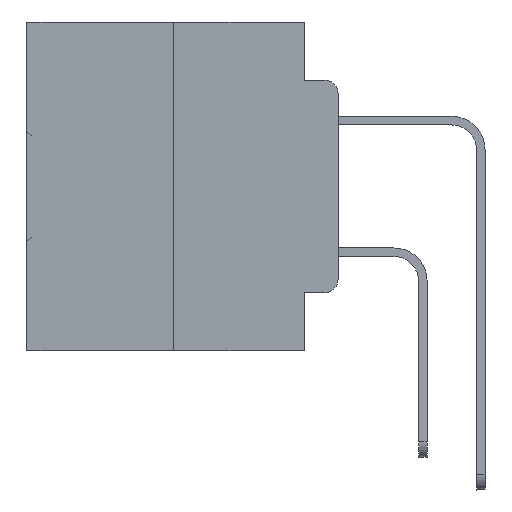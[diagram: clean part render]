
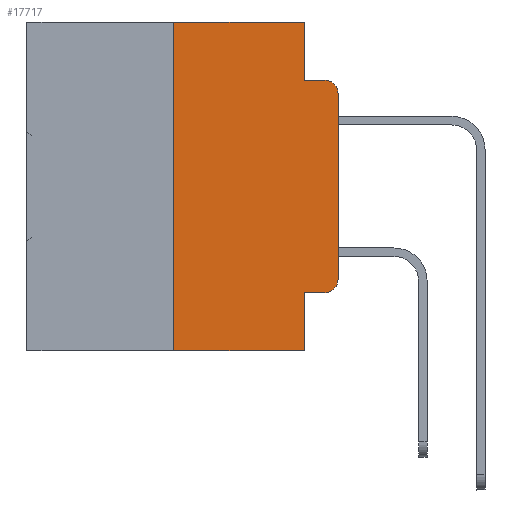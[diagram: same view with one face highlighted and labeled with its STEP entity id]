
A CAD part, left-side view. The second image highlights one B-rep face of the part: STEP entity #17717.
In plain terms, the highlighted planar face has unit normal (-1, 0, 0).
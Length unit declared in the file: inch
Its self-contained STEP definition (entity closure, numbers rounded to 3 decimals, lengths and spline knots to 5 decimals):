
#127 = CARTESIAN_POINT ( 'NONE',  ( 0., 0., -0.1085 ) ) ;
#275 = CARTESIAN_POINT ( 'NONE',  ( 0., 0., -0.3915 ) ) ;
#733 = VERTEX_POINT ( 'NONE', #14793 ) ;
#1035 = EDGE_CURVE ( 'NONE', #28705, #18398, #30167, .T. ) ;
#1122 = CARTESIAN_POINT ( 'NONE',  ( 0., 0.02, -0.4115 ) ) ;
#2019 = ORIENTED_EDGE ( 'NONE', *, *, #21079, .T. ) ;
#2238 = DIRECTION ( 'NONE',  ( 0., -1., 0. ) ) ;
#2484 = CARTESIAN_POINT ( 'NONE',  ( 0., 0.051, -0.4115 ) ) ;
#2730 = DIRECTION ( 'NONE',  ( 0., 0., -1. ) ) ;
#3255 = EDGE_CURVE ( 'NONE', #33308, #11159, #5684, .T. ) ;
#3441 = VERTEX_POINT ( 'NONE', #275 ) ;
#3727 = EDGE_CURVE ( 'NONE', #733, #33305, #19545, .T. ) ;
#3817 = VERTEX_POINT ( 'NONE', #9020 ) ;
#4378 = DIRECTION ( 'NONE',  ( 0., 0., 1. ) ) ;
#4579 = VECTOR ( 'NONE', #25150, 39.37008 ) ;
#4669 = DIRECTION ( 'NONE',  ( 0., -1., 0. ) ) ;
#4711 = ORIENTED_EDGE ( 'NONE', *, *, #23275, .F. ) ;
#5159 = VECTOR ( 'NONE', #10803, 39.37008 ) ;
#5537 = ORIENTED_EDGE ( 'NONE', *, *, #3255, .F. ) ;
#5684 = LINE ( 'NONE', #8152, #5159 ) ;
#6364 = CARTESIAN_POINT ( 'NONE',  ( 0., 0., 0. ) ) ;
#6912 = ORIENTED_EDGE ( 'NONE', *, *, #14111, .T. ) ;
#7627 = CARTESIAN_POINT ( 'NONE',  ( 0., 0.051, -0.5 ) ) ;
#8152 = CARTESIAN_POINT ( 'NONE',  ( 0., 0.051, 0. ) ) ;
#8409 = AXIS2_PLACEMENT_3D ( 'NONE', #15886, #36053, #30482 ) ;
#8677 = DIRECTION ( 'NONE',  ( 1., 0., 0. ) ) ;
#9020 = CARTESIAN_POINT ( 'NONE',  ( 0., 0.02, -0.0885 ) ) ;
#9132 = VERTEX_POINT ( 'NONE', #127 ) ;
#9646 = VECTOR ( 'NONE', #20025, 39.37008 ) ;
#9739 = CIRCLE ( 'NONE', #19317, 0.02 ) ;
#10653 = CARTESIAN_POINT ( 'NONE',  ( 0., 0.25, 0. ) ) ;
#10803 = DIRECTION ( 'NONE',  ( 0., 0., -1. ) ) ;
#11159 = VERTEX_POINT ( 'NONE', #26830 ) ;
#11450 = AXIS2_PLACEMENT_3D ( 'NONE', #17324, #8677, #31717 ) ;
#12255 = ORIENTED_EDGE ( 'NONE', *, *, #18828, .F. ) ;
#12570 = CARTESIAN_POINT ( 'NONE',  ( 0., 0.051, 0. ) ) ;
#12700 = ORIENTED_EDGE ( 'NONE', *, *, #20068, .F. ) ;
#12758 = ORIENTED_EDGE ( 'NONE', *, *, #30528, .F. ) ;
#12812 = ORIENTED_EDGE ( 'NONE', *, *, #3727, .T. ) ;
#12979 = CARTESIAN_POINT ( 'NONE',  ( 0., 0.25, -0.5 ) ) ;
#14111 = EDGE_CURVE ( 'NONE', #3441, #9132, #20619, .T. ) ;
#14793 = CARTESIAN_POINT ( 'NONE',  ( 0., 0.051, -0.4115 ) ) ;
#15175 = EDGE_LOOP ( 'NONE', ( #6912, #30542, #12255, #5537, #4711, #12700, #18492, #12758, #12812, #2019 ) ) ;
#15388 = DIRECTION ( 'NONE',  ( 0., 0., 1. ) ) ;
#15426 = VECTOR ( 'NONE', #4669, 39.37008 ) ;
#15886 = CARTESIAN_POINT ( 'NONE',  ( 0., 0.02, -0.1085 ) ) ;
#15957 = CARTESIAN_POINT ( 'NONE',  ( 0., 0.473, -0.5 ) ) ;
#17238 = LINE ( 'NONE', #19160, #9646 ) ;
#17324 = CARTESIAN_POINT ( 'NONE',  ( 0., 0.473, 0. ) ) ;
#17368 = DIRECTION ( 'NONE',  ( -1., 0., 0. ) ) ;
#17717 = ADVANCED_FACE ( 'NONE', ( #23096 ), #36930, .F. ) ;
#18398 = VERTEX_POINT ( 'NONE', #7627 ) ;
#18492 = ORIENTED_EDGE ( 'NONE', *, *, #1035, .T. ) ;
#18828 = EDGE_CURVE ( 'NONE', #11159, #3817, #24083, .T. ) ;
#18838 = CARTESIAN_POINT ( 'NONE',  ( 0., 0.25, 0. ) ) ;
#19160 = CARTESIAN_POINT ( 'NONE',  ( 0., 0.051, 0. ) ) ;
#19317 = AXIS2_PLACEMENT_3D ( 'NONE', #33830, #17368, #2730 ) ;
#19545 = LINE ( 'NONE', #2484, #4579 ) ;
#20025 = DIRECTION ( 'NONE',  ( 0., 0., -1. ) ) ;
#20068 = EDGE_CURVE ( 'NONE', #28705, #30842, #21646, .T. ) ;
#20619 = LINE ( 'NONE', #6364, #34555 ) ;
#21079 = EDGE_CURVE ( 'NONE', #33305, #3441, #9739, .T. ) ;
#21646 = LINE ( 'NONE', #18838, #22272 ) ;
#21852 = VECTOR ( 'NONE', #2238, 39.37008 ) ;
#22272 = VECTOR ( 'NONE', #4378, 39.37008 ) ;
#23096 = FACE_OUTER_BOUND ( 'NONE', #15175, .T. ) ;
#23275 = EDGE_CURVE ( 'NONE', #30842, #33308, #33880, .T. ) ;
#23336 = VECTOR ( 'NONE', #33251, 39.37008 ) ;
#23344 = CIRCLE ( 'NONE', #8409, 0.02 ) ;
#24083 = LINE ( 'NONE', #35474, #23336 ) ;
#25150 = DIRECTION ( 'NONE',  ( 0., -1., 0. ) ) ;
#26830 = CARTESIAN_POINT ( 'NONE',  ( 0., 0.051, -0.0885 ) ) ;
#28241 = EDGE_CURVE ( 'NONE', #9132, #3817, #23344, .T. ) ;
#28705 = VERTEX_POINT ( 'NONE', #12979 ) ;
#30167 = LINE ( 'NONE', #15957, #15426 ) ;
#30482 = DIRECTION ( 'NONE',  ( 0., 0., -1. ) ) ;
#30528 = EDGE_CURVE ( 'NONE', #733, #18398, #17238, .T. ) ;
#30542 = ORIENTED_EDGE ( 'NONE', *, *, #28241, .T. ) ;
#30842 = VERTEX_POINT ( 'NONE', #10653 ) ;
#31717 = DIRECTION ( 'NONE',  ( 0., 0., -1. ) ) ;
#33251 = DIRECTION ( 'NONE',  ( 0., -1., 0. ) ) ;
#33305 = VERTEX_POINT ( 'NONE', #1122 ) ;
#33308 = VERTEX_POINT ( 'NONE', #12570 ) ;
#33338 = CARTESIAN_POINT ( 'NONE',  ( 0., 0.473, 0. ) ) ;
#33830 = CARTESIAN_POINT ( 'NONE',  ( 0., 0.02, -0.3915 ) ) ;
#33880 = LINE ( 'NONE', #33338, #21852 ) ;
#34555 = VECTOR ( 'NONE', #15388, 39.37008 ) ;
#35474 = CARTESIAN_POINT ( 'NONE',  ( 0., 0.051, -0.0885 ) ) ;
#36053 = DIRECTION ( 'NONE',  ( -1., 0., 0. ) ) ;
#36930 = PLANE ( 'NONE',  #11450 ) ;
